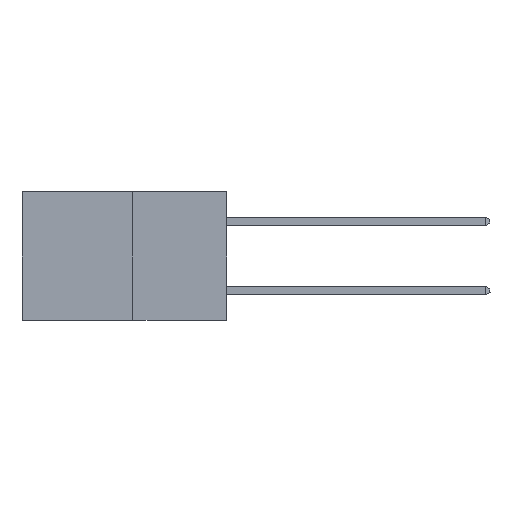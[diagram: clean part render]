
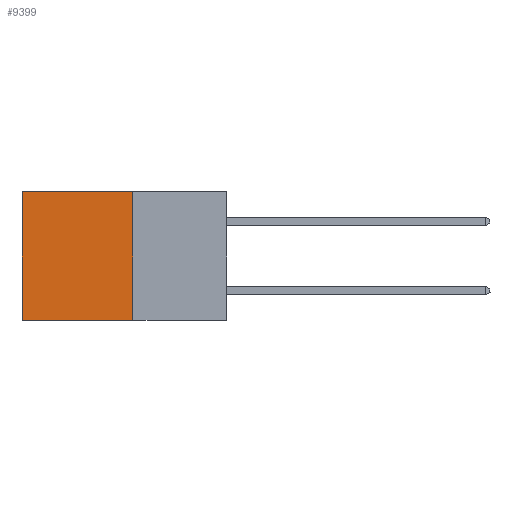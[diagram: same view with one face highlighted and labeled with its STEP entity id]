
A CAD part, left-side view. The second image highlights one B-rep face of the part: STEP entity #9399.
In plain terms, the highlighted planar face has unit normal (-1, 0, 0).
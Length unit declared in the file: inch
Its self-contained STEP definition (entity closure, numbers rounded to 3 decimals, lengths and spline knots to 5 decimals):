
#382 = CARTESIAN_POINT ( 'NONE',  ( 0.277, 0.27, -0.37 ) ) ;
#2042 = VECTOR ( 'NONE', #21473, 39.37008 ) ;
#2232 = DIRECTION ( 'NONE',  ( 0., 0., -1. ) ) ;
#2480 = CARTESIAN_POINT ( 'NONE',  ( 0.277, 0.27, 0. ) ) ;
#2962 = LINE ( 'NONE', #2480, #12045 ) ;
#3484 = EDGE_CURVE ( 'NONE', #5222, #12656, #5136, .T. ) ;
#4287 = DIRECTION ( 'NONE',  ( 0., 1., 0. ) ) ;
#4697 = EDGE_CURVE ( 'NONE', #12656, #22444, #21208, .T. ) ;
#5136 = LINE ( 'NONE', #8089, #9386 ) ;
#5222 = VERTEX_POINT ( 'NONE', #10436 ) ;
#6655 = AXIS2_PLACEMENT_3D ( 'NONE', #382, #13075, #2232 ) ;
#7508 = EDGE_CURVE ( 'NONE', #16094, #22444, #14956, .T. ) ;
#8089 = CARTESIAN_POINT ( 'NONE',  ( 0.277, 0.27, -0.37 ) ) ;
#8334 = CARTESIAN_POINT ( 'NONE',  ( 0.277, 0.59, 0. ) ) ;
#9147 = ORIENTED_EDGE ( 'NONE', *, *, #4697, .F. ) ;
#9386 = VECTOR ( 'NONE', #9783, 39.37008 ) ;
#9399 = ADVANCED_FACE ( 'NONE', ( #12058 ), #18408, .F. ) ;
#9783 = DIRECTION ( 'NONE',  ( 0., 0., -1. ) ) ;
#10132 = ORIENTED_EDGE ( 'NONE', *, *, #7508, .T. ) ;
#10436 = CARTESIAN_POINT ( 'NONE',  ( 0.277, 0.27, 0. ) ) ;
#10924 = EDGE_CURVE ( 'NONE', #5222, #16094, #2962, .T. ) ;
#12045 = VECTOR ( 'NONE', #4287, 39.37008 ) ;
#12058 = FACE_OUTER_BOUND ( 'NONE', #20898, .T. ) ;
#12656 = VERTEX_POINT ( 'NONE', #13402 ) ;
#13075 = DIRECTION ( 'NONE',  ( 1., 0., 0. ) ) ;
#13402 = CARTESIAN_POINT ( 'NONE',  ( 0.277, 0.27, -0.37 ) ) ;
#14394 = VECTOR ( 'NONE', #21998, 39.37008 ) ;
#14956 = LINE ( 'NONE', #20211, #14394 ) ;
#15777 = ORIENTED_EDGE ( 'NONE', *, *, #10924, .T. ) ;
#16094 = VERTEX_POINT ( 'NONE', #8334 ) ;
#18408 = PLANE ( 'NONE',  #6655 ) ;
#20211 = CARTESIAN_POINT ( 'NONE',  ( 0.277, 0.59, -0.37 ) ) ;
#20247 = ORIENTED_EDGE ( 'NONE', *, *, #3484, .F. ) ;
#20824 = CARTESIAN_POINT ( 'NONE',  ( 0.277, 0.59, -0.37 ) ) ;
#20898 = EDGE_LOOP ( 'NONE', ( #10132, #9147, #20247, #15777 ) ) ;
#21208 = LINE ( 'NONE', #23003, #2042 ) ;
#21473 = DIRECTION ( 'NONE',  ( 0., 1., 0. ) ) ;
#21998 = DIRECTION ( 'NONE',  ( 0., 0., -1. ) ) ;
#22444 = VERTEX_POINT ( 'NONE', #20824 ) ;
#23003 = CARTESIAN_POINT ( 'NONE',  ( 0.277, 0.27, -0.37 ) ) ;
